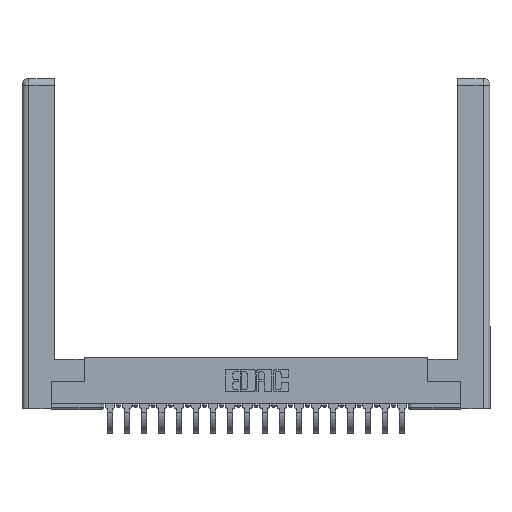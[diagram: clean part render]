
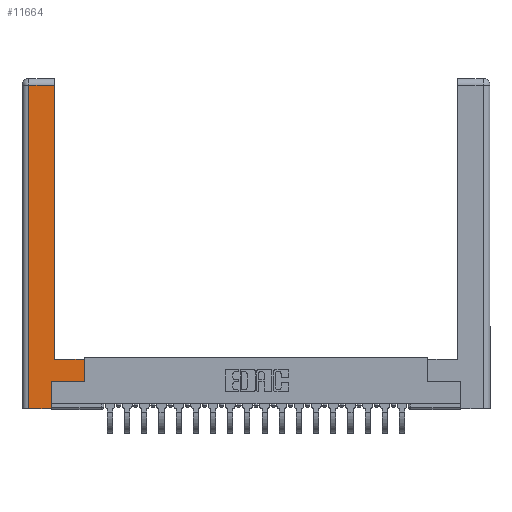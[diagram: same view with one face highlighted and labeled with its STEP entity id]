
A CAD part, top view. The second image highlights one B-rep face of the part: STEP entity #11664.
In plain terms, the highlighted planar face has unit normal (0, 0, 1).
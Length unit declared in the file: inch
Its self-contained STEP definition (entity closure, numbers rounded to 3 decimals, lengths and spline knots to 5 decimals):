
#29 = LINE ( 'NONE', #4013, #4046 ) ;
#279 = DIRECTION ( 'NONE',  ( -1., 0., 0. ) ) ;
#613 = DIRECTION ( 'NONE',  ( 0., 1., 0. ) ) ;
#1019 = CARTESIAN_POINT ( 'NONE',  ( 0.265, 0., 0. ) ) ;
#1039 = CARTESIAN_POINT ( 'NONE',  ( 0.265, 0.245, 0. ) ) ;
#1377 = VECTOR ( 'NONE', #19050, 39.37008 ) ;
#2278 = LINE ( 'NONE', #21883, #17492 ) ;
#2346 = VERTEX_POINT ( 'NONE', #1019 ) ;
#2485 = VERTEX_POINT ( 'NONE', #20632 ) ;
#3293 = ORIENTED_EDGE ( 'NONE', *, *, #21996, .T. ) ;
#3547 = ORIENTED_EDGE ( 'NONE', *, *, #16456, .T. ) ;
#4013 = CARTESIAN_POINT ( 'NONE',  ( 0.565, 0.45, 0. ) ) ;
#4046 = VECTOR ( 'NONE', #613, 39.37008 ) ;
#4283 = ORIENTED_EDGE ( 'NONE', *, *, #10186, .T. ) ;
#4908 = FACE_OUTER_BOUND ( 'NONE', #10432, .T. ) ;
#5203 = ORIENTED_EDGE ( 'NONE', *, *, #20295, .T. ) ;
#5376 = CARTESIAN_POINT ( 'NONE',  ( 0.0615, 0., 0. ) ) ;
#5469 = VERTEX_POINT ( 'NONE', #21818 ) ;
#5614 = VERTEX_POINT ( 'NONE', #1039 ) ;
#5839 = CARTESIAN_POINT ( 'NONE',  ( 0.0615, 2.94, 0. ) ) ;
#6086 = DIRECTION ( 'NONE',  ( 1., 0., 0. ) ) ;
#6746 = ORIENTED_EDGE ( 'NONE', *, *, #20790, .T. ) ;
#7938 = EDGE_CURVE ( 'NONE', #2485, #18580, #29, .T. ) ;
#8388 = AXIS2_PLACEMENT_3D ( 'NONE', #13676, #13796, #19141 ) ;
#8945 = CARTESIAN_POINT ( 'NONE',  ( 0.295, 0.45, 0. ) ) ;
#9611 = LINE ( 'NONE', #14971, #22087 ) ;
#9865 = EDGE_CURVE ( 'NONE', #2346, #5614, #9611, .T. ) ;
#10186 = EDGE_CURVE ( 'NONE', #16319, #2346, #14837, .T. ) ;
#10432 = EDGE_LOOP ( 'NONE', ( #3293, #3547, #14794, #4283, #20233, #6746, #13367, #5203 ) ) ;
#10804 = LINE ( 'NONE', #8945, #22948 ) ;
#11192 = LINE ( 'NONE', #5839, #17089 ) ;
#11664 = ADVANCED_FACE ( 'NONE', ( #4908 ), #22524, .F. ) ;
#12921 = CARTESIAN_POINT ( 'NONE',  ( 0.0615, 2.94, 0. ) ) ;
#13232 = DIRECTION ( 'NONE',  ( 0., 1., 0. ) ) ;
#13348 = CARTESIAN_POINT ( 'NONE',  ( 0.295, 3., 0. ) ) ;
#13367 = ORIENTED_EDGE ( 'NONE', *, *, #7938, .T. ) ;
#13676 = CARTESIAN_POINT ( 'NONE',  ( 0., 0., 0. ) ) ;
#13796 = DIRECTION ( 'NONE',  ( 0., 0., -1. ) ) ;
#14702 = DIRECTION ( 'NONE',  ( -1., 0., 0. ) ) ;
#14794 = ORIENTED_EDGE ( 'NONE', *, *, #17578, .T. ) ;
#14837 = LINE ( 'NONE', #20085, #19119 ) ;
#14864 = LINE ( 'NONE', #13348, #1377 ) ;
#14971 = CARTESIAN_POINT ( 'NONE',  ( 0.265, 0.245, 0. ) ) ;
#16273 = VECTOR ( 'NONE', #17995, 39.37008 ) ;
#16319 = VERTEX_POINT ( 'NONE', #5376 ) ;
#16380 = CARTESIAN_POINT ( 'NONE',  ( 0.565, 0.245, 0. ) ) ;
#16456 = EDGE_CURVE ( 'NONE', #21610, #17500, #11192, .T. ) ;
#17089 = VECTOR ( 'NONE', #14702, 39.37008 ) ;
#17492 = VECTOR ( 'NONE', #22232, 39.37008 ) ;
#17500 = VERTEX_POINT ( 'NONE', #12921 ) ;
#17578 = EDGE_CURVE ( 'NONE', #17500, #16319, #2278, .T. ) ;
#17995 = DIRECTION ( 'NONE',  ( 1., 0., 0. ) ) ;
#18118 = LINE ( 'NONE', #16380, #16273 ) ;
#18580 = VERTEX_POINT ( 'NONE', #22617 ) ;
#19050 = DIRECTION ( 'NONE',  ( 0., 1., 0. ) ) ;
#19119 = VECTOR ( 'NONE', #6086, 39.37008 ) ;
#19141 = DIRECTION ( 'NONE',  ( -1., 0., 0. ) ) ;
#20085 = CARTESIAN_POINT ( 'NONE',  ( 0.265, 0., 0. ) ) ;
#20233 = ORIENTED_EDGE ( 'NONE', *, *, #9865, .T. ) ;
#20295 = EDGE_CURVE ( 'NONE', #18580, #5469, #10804, .T. ) ;
#20632 = CARTESIAN_POINT ( 'NONE',  ( 0.565, 0.245, 0. ) ) ;
#20790 = EDGE_CURVE ( 'NONE', #5614, #2485, #18118, .T. ) ;
#21610 = VERTEX_POINT ( 'NONE', #22693 ) ;
#21818 = CARTESIAN_POINT ( 'NONE',  ( 0.295, 0.45, 0. ) ) ;
#21883 = CARTESIAN_POINT ( 'NONE',  ( 0.0615, 0., 0. ) ) ;
#21996 = EDGE_CURVE ( 'NONE', #5469, #21610, #14864, .T. ) ;
#22087 = VECTOR ( 'NONE', #13232, 39.37008 ) ;
#22232 = DIRECTION ( 'NONE',  ( 0., -1., 0. ) ) ;
#22524 = PLANE ( 'NONE',  #8388 ) ;
#22617 = CARTESIAN_POINT ( 'NONE',  ( 0.565, 0.45, 0. ) ) ;
#22693 = CARTESIAN_POINT ( 'NONE',  ( 0.295, 2.94, 0. ) ) ;
#22948 = VECTOR ( 'NONE', #279, 39.37008 ) ;
